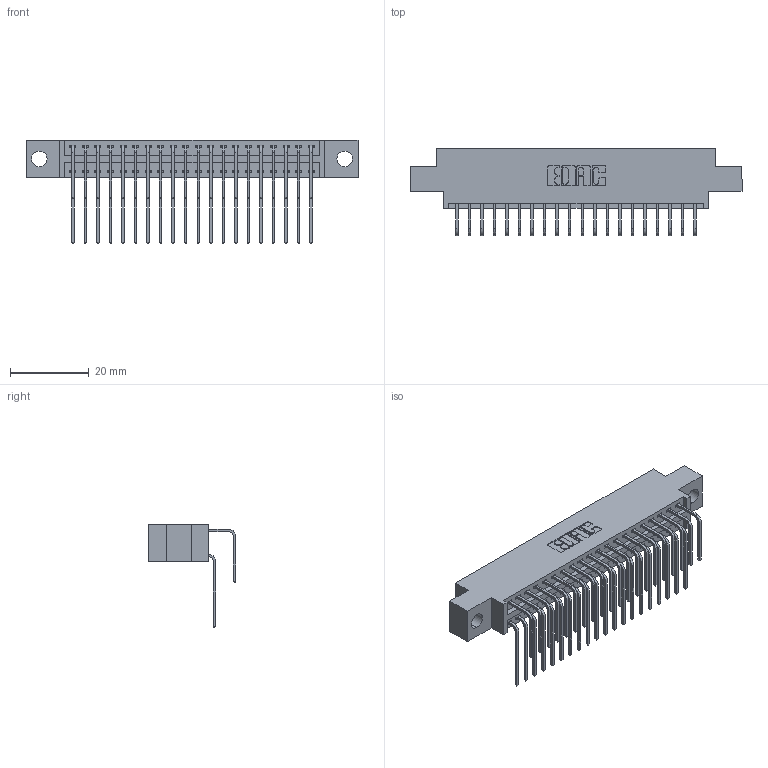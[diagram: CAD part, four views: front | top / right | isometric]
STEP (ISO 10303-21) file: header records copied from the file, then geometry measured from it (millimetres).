
FILE_DESCRIPTION (( 'STEP AP203' ), '1' );
FILE_NAME ('346-040-558-804.STEP', '2022-05-20T02:52:23', ( '' ), ( '' ), 'SwSTEP 2.0', 'SolidWorks 2020', '' );
FILE_SCHEMA (( 'CONFIG_CONTROL_DESIGN' ));
Length unit declared in the file: inch
Products named in the file (4): 346-040-558-804; 345-292-001_558 Tail - 2; 346 Part_0.170 Offset - 0.156 Dia-TH; 345-292-001_558 559 Tail - 1
Assembly tree (41 placements, depth 2):
  346-040-558-804
    346 Part_0.170 Offset - 0.156 Dia-TH
    345-292-001_558 559 Tail - 1  x20
    345-292-001_558 Tail - 2  x20
Bounding box: 84.07 x 22.16 x 26.16 mm (x, y, z)
Volume: 7997.6 mm3; surface area: 11781.9 mm2
Topology: 41 solids, 41 shells, 2300 faces, 6817 edges, 4490 vertices
Faces by surface type: plane 1574, cylinder 726
Entity records: 18349 total; most frequent: CARTESIAN_POINT 3113, ORIENTED_EDGE 2994, DIRECTION 2765, EDGE_CURVE 1497, LINE 1245, VECTOR 1245, VERTEX_POINT 994, AXIS2_PLACEMENT_3D 760
